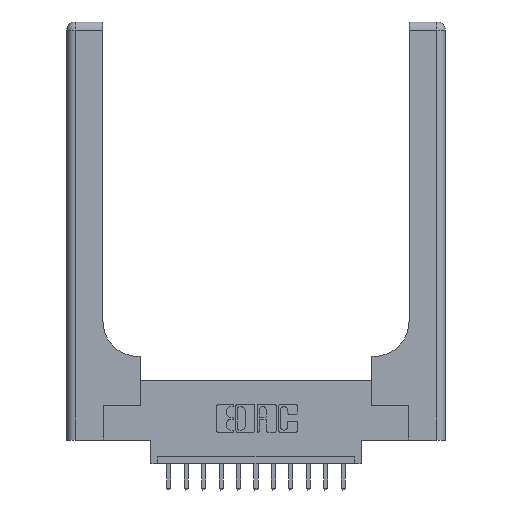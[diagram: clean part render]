
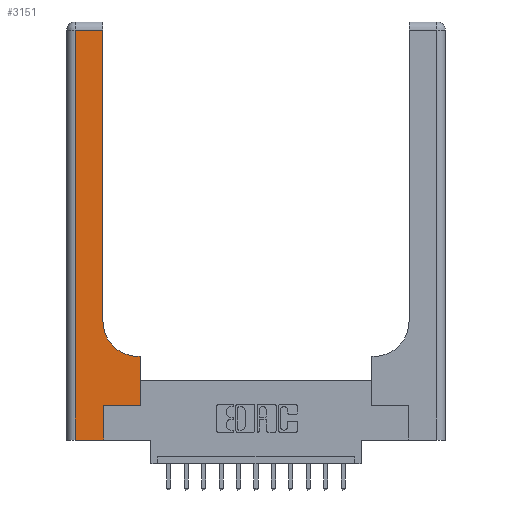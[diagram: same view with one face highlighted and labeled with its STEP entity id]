
A CAD part, top view. The second image highlights one B-rep face of the part: STEP entity #3151.
In plain terms, the highlighted planar face has unit normal (0, 0, 1).
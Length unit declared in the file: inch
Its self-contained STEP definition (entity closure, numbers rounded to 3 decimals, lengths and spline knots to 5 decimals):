
#94 = ORIENTED_EDGE ( 'NONE', *, *, #8680, .T. ) ;
#153 = CARTESIAN_POINT ( 'NONE',  ( 0.26, 0.6, 0.37 ) ) ;
#221 = LINE ( 'NONE', #9995, #11345 ) ;
#319 = VERTEX_POINT ( 'NONE', #3726 ) ;
#627 = DIRECTION ( 'NONE',  ( 0., 1., 0. ) ) ;
#725 = VERTEX_POINT ( 'NONE', #12524 ) ;
#825 = ORIENTED_EDGE ( 'NONE', *, *, #9555, .T. ) ;
#1000 = DIRECTION ( 'NONE',  ( 1., 0., 0. ) ) ;
#1454 = EDGE_CURVE ( 'NONE', #4338, #16381, #12581, .T. ) ;
#1530 = ORIENTED_EDGE ( 'NONE', *, *, #8544, .T. ) ;
#1602 = DIRECTION ( 'NONE',  ( 0., 0., -1. ) ) ;
#1620 = CARTESIAN_POINT ( 'NONE',  ( 0.265, 0.25, 0.37 ) ) ;
#1976 = EDGE_CURVE ( 'NONE', #725, #14035, #15314, .T. ) ;
#2055 = VECTOR ( 'NONE', #627, 39.37008 ) ;
#2172 = ORIENTED_EDGE ( 'NONE', *, *, #8038, .T. ) ;
#2369 = DIRECTION ( 'NONE',  ( 0., -1., 0. ) ) ;
#2734 = DIRECTION ( 'NONE',  ( -1., 0., 0. ) ) ;
#2797 = LINE ( 'NONE', #15505, #15893 ) ;
#2915 = DIRECTION ( 'NONE',  ( -1., 0., 0. ) ) ;
#3151 = ADVANCED_FACE ( 'NONE', ( #11131 ), #14239, .F. ) ;
#3588 = CIRCLE ( 'NONE', #5402, 0.25 ) ;
#3639 = ORIENTED_EDGE ( 'NONE', *, *, #1454, .T. ) ;
#3726 = CARTESIAN_POINT ( 'NONE',  ( 0.51, 0.6, 0.37 ) ) ;
#3732 = EDGE_LOOP ( 'NONE', ( #825, #3639, #94, #2172, #7700, #5151, #5743, #15028, #1530 ) ) ;
#4338 = VERTEX_POINT ( 'NONE', #11005 ) ;
#5151 = ORIENTED_EDGE ( 'NONE', *, *, #14387, .T. ) ;
#5402 = AXIS2_PLACEMENT_3D ( 'NONE', #8011, #1602, #10420 ) ;
#5743 = ORIENTED_EDGE ( 'NONE', *, *, #13564, .T. ) ;
#5795 = EDGE_CURVE ( 'NONE', #13540, #319, #14733, .T. ) ;
#5945 = VECTOR ( 'NONE', #10545, 39.37008 ) ;
#6386 = CARTESIAN_POINT ( 'NONE',  ( 0.06, 0., 0.37 ) ) ;
#6411 = LINE ( 'NONE', #7432, #16098 ) ;
#7432 = CARTESIAN_POINT ( 'NONE',  ( 0.06, 3., 0.37 ) ) ;
#7700 = ORIENTED_EDGE ( 'NONE', *, *, #1976, .T. ) ;
#7832 = CARTESIAN_POINT ( 'NONE',  ( 0.528, 0.25, 0.37 ) ) ;
#7951 = DIRECTION ( 'NONE',  ( 0., 1., 0. ) ) ;
#8011 = CARTESIAN_POINT ( 'NONE',  ( 0.51, 0.85, 0.37 ) ) ;
#8038 = EDGE_CURVE ( 'NONE', #11584, #725, #221, .T. ) ;
#8457 = DIRECTION ( 'NONE',  ( 0., 1., 0. ) ) ;
#8544 = EDGE_CURVE ( 'NONE', #319, #11101, #3588, .T. ) ;
#8680 = EDGE_CURVE ( 'NONE', #16381, #11584, #6411, .T. ) ;
#9069 = CARTESIAN_POINT ( 'NONE',  ( 0., 2.94, 0.37 ) ) ;
#9213 = VECTOR ( 'NONE', #12717, 39.37008 ) ;
#9555 = EDGE_CURVE ( 'NONE', #11101, #4338, #2797, .T. ) ;
#9995 = CARTESIAN_POINT ( 'NONE',  ( 0., 0., 0.37 ) ) ;
#10420 = DIRECTION ( 'NONE',  ( 1., 0., 0. ) ) ;
#10505 = CARTESIAN_POINT ( 'NONE',  ( 0., 3., 0.37 ) ) ;
#10545 = DIRECTION ( 'NONE',  ( 1., 0., 0. ) ) ;
#10943 = VERTEX_POINT ( 'NONE', #7832 ) ;
#11005 = CARTESIAN_POINT ( 'NONE',  ( 0.26, 2.94, 0.37 ) ) ;
#11101 = VERTEX_POINT ( 'NONE', #12382 ) ;
#11131 = FACE_OUTER_BOUND ( 'NONE', #3732, .T. ) ;
#11345 = VECTOR ( 'NONE', #1000, 39.37008 ) ;
#11584 = VERTEX_POINT ( 'NONE', #6386 ) ;
#11840 = DIRECTION ( 'NONE',  ( 0., 0., -1. ) ) ;
#12139 = CARTESIAN_POINT ( 'NONE',  ( 0.265, 0., 0.37 ) ) ;
#12382 = CARTESIAN_POINT ( 'NONE',  ( 0.26, 0.85, 0.37 ) ) ;
#12524 = CARTESIAN_POINT ( 'NONE',  ( 0.265, 0., 0.37 ) ) ;
#12581 = LINE ( 'NONE', #9069, #9213 ) ;
#12636 = LINE ( 'NONE', #1620, #5945 ) ;
#12717 = DIRECTION ( 'NONE',  ( -1., 0., 0. ) ) ;
#12853 = VECTOR ( 'NONE', #8457, 39.37008 ) ;
#13016 = CARTESIAN_POINT ( 'NONE',  ( 0.265, 0.25, 0.37 ) ) ;
#13040 = LINE ( 'NONE', #15986, #12853 ) ;
#13254 = CARTESIAN_POINT ( 'NONE',  ( 0.528, 0.6, 0.37 ) ) ;
#13540 = VERTEX_POINT ( 'NONE', #13254 ) ;
#13564 = EDGE_CURVE ( 'NONE', #10943, #13540, #13040, .T. ) ;
#13776 = AXIS2_PLACEMENT_3D ( 'NONE', #10505, #11840, #2915 ) ;
#13783 = CARTESIAN_POINT ( 'NONE',  ( 0.06, 2.94, 0.37 ) ) ;
#14035 = VERTEX_POINT ( 'NONE', #13016 ) ;
#14239 = PLANE ( 'NONE',  #13776 ) ;
#14387 = EDGE_CURVE ( 'NONE', #14035, #10943, #12636, .T. ) ;
#14733 = LINE ( 'NONE', #153, #15774 ) ;
#15028 = ORIENTED_EDGE ( 'NONE', *, *, #5795, .T. ) ;
#15314 = LINE ( 'NONE', #12139, #2055 ) ;
#15505 = CARTESIAN_POINT ( 'NONE',  ( 0.26, 3., 0.37 ) ) ;
#15774 = VECTOR ( 'NONE', #2734, 39.37008 ) ;
#15893 = VECTOR ( 'NONE', #7951, 39.37008 ) ;
#15986 = CARTESIAN_POINT ( 'NONE',  ( 0.528, 0.25, 0.37 ) ) ;
#16098 = VECTOR ( 'NONE', #2369, 39.37008 ) ;
#16381 = VERTEX_POINT ( 'NONE', #13783 ) ;
